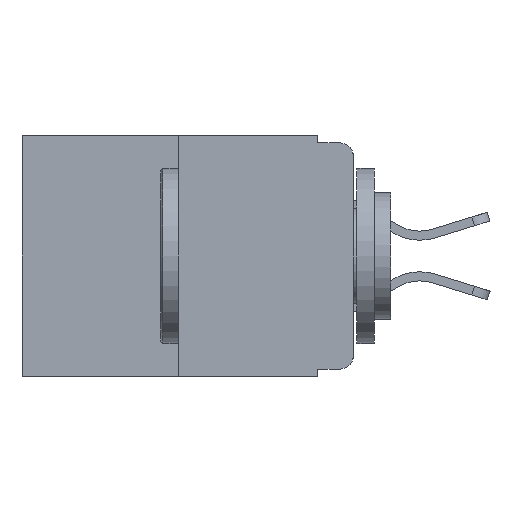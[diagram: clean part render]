
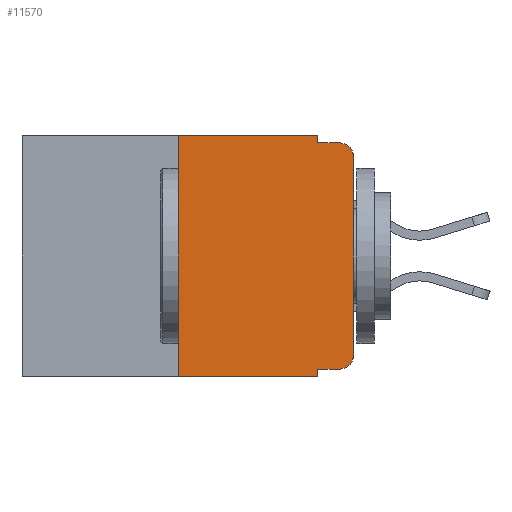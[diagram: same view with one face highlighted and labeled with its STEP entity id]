
A CAD part, left-side view. The second image highlights one B-rep face of the part: STEP entity #11570.
In plain terms, the highlighted planar face has unit normal (-1, 0, 0).
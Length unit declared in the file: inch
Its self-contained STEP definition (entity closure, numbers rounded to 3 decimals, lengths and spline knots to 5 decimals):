
#17 = VECTOR ( 'NONE', #20308, 39.37008 ) ;
#172 = ORIENTED_EDGE ( 'NONE', *, *, #12523, .F. ) ;
#619 = CARTESIAN_POINT ( 'NONE',  ( 0., 0.25, 0. ) ) ;
#700 = DIRECTION ( 'NONE',  ( 0., 0., -1. ) ) ;
#1020 = AXIS2_PLACEMENT_3D ( 'NONE', #17279, #9137, #10916 ) ;
#1234 = LINE ( 'NONE', #20405, #10514 ) ;
#1346 = CARTESIAN_POINT ( 'NONE',  ( 0., 0.473, -0.343 ) ) ;
#2015 = LINE ( 'NONE', #8472, #7109 ) ;
#2370 = CARTESIAN_POINT ( 'NONE',  ( 0., 0.473, 0. ) ) ;
#2835 = EDGE_CURVE ( 'NONE', #3189, #5738, #11644, .T. ) ;
#2923 = DIRECTION ( 'NONE',  ( 0., 0., -1. ) ) ;
#3189 = VERTEX_POINT ( 'NONE', #12503 ) ;
#3283 = VERTEX_POINT ( 'NONE', #9830 ) ;
#3351 = CARTESIAN_POINT ( 'NONE',  ( 0., 0., 0. ) ) ;
#3360 = CARTESIAN_POINT ( 'NONE',  ( 0., 0.25, 0. ) ) ;
#3744 = VECTOR ( 'NONE', #12345, 39.37008 ) ;
#4456 = VERTEX_POINT ( 'NONE', #12506 ) ;
#5063 = AXIS2_PLACEMENT_3D ( 'NONE', #14080, #20559, #17756 ) ;
#5402 = EDGE_CURVE ( 'NONE', #4456, #5738, #9268, .T. ) ;
#5482 = EDGE_CURVE ( 'NONE', #3189, #15720, #1234, .T. ) ;
#5738 = VERTEX_POINT ( 'NONE', #7148 ) ;
#6152 = PLANE ( 'NONE',  #5063 ) ;
#6353 = FACE_OUTER_BOUND ( 'NONE', #10007, .T. ) ;
#6390 = EDGE_CURVE ( 'NONE', #4456, #10960, #11927, .T. ) ;
#6910 = CARTESIAN_POINT ( 'NONE',  ( 0., 0.02, -0.01 ) ) ;
#7109 = VECTOR ( 'NONE', #14915, 39.37008 ) ;
#7148 = CARTESIAN_POINT ( 'NONE',  ( 0., 0.051, -0.343 ) ) ;
#7282 = VERTEX_POINT ( 'NONE', #15035 ) ;
#7470 = VECTOR ( 'NONE', #2923, 39.37008 ) ;
#7893 = ORIENTED_EDGE ( 'NONE', *, *, #5402, .T. ) ;
#8213 = ORIENTED_EDGE ( 'NONE', *, *, #11821, .F. ) ;
#8472 = CARTESIAN_POINT ( 'NONE',  ( 0., 0.051, -0.01 ) ) ;
#8478 = AXIS2_PLACEMENT_3D ( 'NONE', #18356, #16978, #700 ) ;
#8833 = LINE ( 'NONE', #2370, #20286 ) ;
#9137 = DIRECTION ( 'NONE',  ( -1., 0., 0. ) ) ;
#9268 = LINE ( 'NONE', #1346, #3744 ) ;
#9830 = CARTESIAN_POINT ( 'NONE',  ( 0., 0., -0.03 ) ) ;
#9896 = EDGE_CURVE ( 'NONE', #10960, #7282, #8833, .T. ) ;
#9987 = EDGE_CURVE ( 'NONE', #3283, #19104, #13520, .T. ) ;
#10007 = EDGE_LOOP ( 'NONE', ( #12774, #10824, #8213, #172, #10320, #11806, #7893, #17606, #15487, #16986 ) ) ;
#10320 = ORIENTED_EDGE ( 'NONE', *, *, #9896, .F. ) ;
#10514 = VECTOR ( 'NONE', #12453, 39.37008 ) ;
#10739 = VECTOR ( 'NONE', #16447, 39.37008 ) ;
#10824 = ORIENTED_EDGE ( 'NONE', *, *, #9987, .T. ) ;
#10863 = LINE ( 'NONE', #15918, #7470 ) ;
#10916 = DIRECTION ( 'NONE',  ( 0., 0., -1. ) ) ;
#10960 = VERTEX_POINT ( 'NONE', #3360 ) ;
#11548 = CARTESIAN_POINT ( 'NONE',  ( 0., 0.051, 0. ) ) ;
#11570 = ADVANCED_FACE ( 'NONE', ( #6353 ), #6152, .F. ) ;
#11644 = LINE ( 'NONE', #11548, #15763 ) ;
#11806 = ORIENTED_EDGE ( 'NONE', *, *, #6390, .F. ) ;
#11821 = EDGE_CURVE ( 'NONE', #11990, #19104, #2015, .T. ) ;
#11927 = LINE ( 'NONE', #619, #17 ) ;
#11990 = VERTEX_POINT ( 'NONE', #17134 ) ;
#12114 = CARTESIAN_POINT ( 'NONE',  ( 0., 0., -0.313 ) ) ;
#12345 = DIRECTION ( 'NONE',  ( 0., -1., 0. ) ) ;
#12453 = DIRECTION ( 'NONE',  ( 0., -1., 0. ) ) ;
#12503 = CARTESIAN_POINT ( 'NONE',  ( 0., 0.051, -0.333 ) ) ;
#12506 = CARTESIAN_POINT ( 'NONE',  ( 0., 0.25, -0.343 ) ) ;
#12523 = EDGE_CURVE ( 'NONE', #7282, #11990, #10863, .T. ) ;
#12739 = CARTESIAN_POINT ( 'NONE',  ( 0., 0.02, -0.333 ) ) ;
#12774 = ORIENTED_EDGE ( 'NONE', *, *, #18324, .T. ) ;
#12919 = EDGE_CURVE ( 'NONE', #15720, #14208, #14224, .T. ) ;
#13520 = CIRCLE ( 'NONE', #1020, 0.02 ) ;
#14080 = CARTESIAN_POINT ( 'NONE',  ( 0., 0.473, 0. ) ) ;
#14208 = VERTEX_POINT ( 'NONE', #12114 ) ;
#14224 = CIRCLE ( 'NONE', #8478, 0.02 ) ;
#14767 = LINE ( 'NONE', #3351, #10739 ) ;
#14915 = DIRECTION ( 'NONE',  ( 0., -1., 0. ) ) ;
#15035 = CARTESIAN_POINT ( 'NONE',  ( 0., 0.051, 0. ) ) ;
#15487 = ORIENTED_EDGE ( 'NONE', *, *, #5482, .T. ) ;
#15720 = VERTEX_POINT ( 'NONE', #12739 ) ;
#15763 = VECTOR ( 'NONE', #17997, 39.37008 ) ;
#15918 = CARTESIAN_POINT ( 'NONE',  ( 0., 0.051, 0. ) ) ;
#16447 = DIRECTION ( 'NONE',  ( 0., 0., 1. ) ) ;
#16978 = DIRECTION ( 'NONE',  ( -1., 0., 0. ) ) ;
#16986 = ORIENTED_EDGE ( 'NONE', *, *, #12919, .T. ) ;
#17134 = CARTESIAN_POINT ( 'NONE',  ( 0., 0.051, -0.01 ) ) ;
#17279 = CARTESIAN_POINT ( 'NONE',  ( 0., 0.02, -0.03 ) ) ;
#17606 = ORIENTED_EDGE ( 'NONE', *, *, #2835, .F. ) ;
#17756 = DIRECTION ( 'NONE',  ( 0., 0., -1. ) ) ;
#17997 = DIRECTION ( 'NONE',  ( 0., 0., -1. ) ) ;
#18324 = EDGE_CURVE ( 'NONE', #14208, #3283, #14767, .T. ) ;
#18356 = CARTESIAN_POINT ( 'NONE',  ( 0., 0.02, -0.313 ) ) ;
#19104 = VERTEX_POINT ( 'NONE', #6910 ) ;
#19179 = DIRECTION ( 'NONE',  ( 0., -1., 0. ) ) ;
#20286 = VECTOR ( 'NONE', #19179, 39.37008 ) ;
#20308 = DIRECTION ( 'NONE',  ( 0., 0., 1. ) ) ;
#20405 = CARTESIAN_POINT ( 'NONE',  ( 0., 0.051, -0.333 ) ) ;
#20559 = DIRECTION ( 'NONE',  ( 1., 0., 0. ) ) ;
